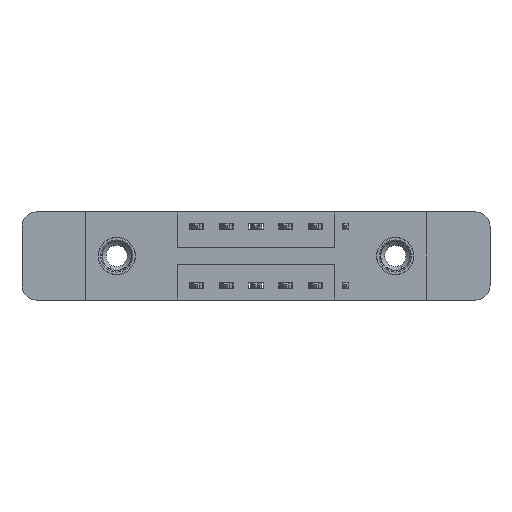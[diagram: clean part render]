
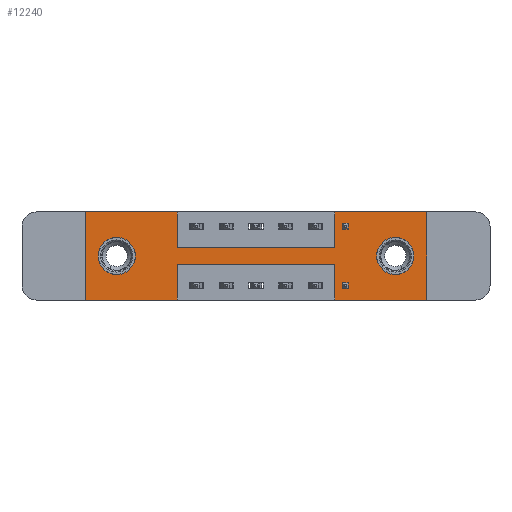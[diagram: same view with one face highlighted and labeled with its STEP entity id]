
A CAD part, front view. The second image highlights one B-rep face of the part: STEP entity #12240.
In plain terms, the highlighted planar face has unit normal (0, -1, 0).
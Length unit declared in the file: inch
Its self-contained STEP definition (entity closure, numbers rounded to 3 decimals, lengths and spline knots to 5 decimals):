
#74 = EDGE_CURVE ( 'NONE', #13054, #4540, #6638, .T. ) ;
#94 = DIRECTION ( 'NONE',  ( 0., 1., 0. ) ) ;
#152 = VECTOR ( 'NONE', #12726, 39.37008 ) ;
#212 = EDGE_CURVE ( 'NONE', #2639, #922, #11114, .T. ) ;
#272 = CARTESIAN_POINT ( 'NONE',  ( 0.1325, 0., -0.185 ) ) ;
#595 = EDGE_CURVE ( 'NONE', #10649, #8934, #3560, .T. ) ;
#611 = CARTESIAN_POINT ( 'NONE',  ( 0., 0., 0. ) ) ;
#614 = VERTEX_POINT ( 'NONE', #12001 ) ;
#895 = VECTOR ( 'NONE', #10591, 39.37008 ) ;
#922 = VERTEX_POINT ( 'NONE', #11918 ) ;
#938 = LINE ( 'NONE', #1008, #13102 ) ;
#957 = ORIENTED_EDGE ( 'NONE', *, *, #212, .F. ) ;
#1008 = CARTESIAN_POINT ( 'NONE',  ( 0., 0., -0.37 ) ) ;
#1032 = CARTESIAN_POINT ( 'NONE',  ( 0., 0., 0. ) ) ;
#1251 = VERTEX_POINT ( 'NONE', #7436 ) ;
#1263 = CARTESIAN_POINT ( 'NONE',  ( 1.3025, 0., -0.107 ) ) ;
#1266 = VECTOR ( 'NONE', #9973, 39.37008 ) ;
#1365 = EDGE_LOOP ( 'NONE', ( #5945, #7739, #6471, #9340, #9083, #13688, #10177, #9714, #957, #5654, #2848, #6998 ) ) ;
#1368 = CARTESIAN_POINT ( 'NONE',  ( 1.0475, 0., -0.37 ) ) ;
#1430 = VECTOR ( 'NONE', #10830, 39.37008 ) ;
#1546 = VERTEX_POINT ( 'NONE', #3613 ) ;
#1588 = LINE ( 'NONE', #611, #12780 ) ;
#1657 = VERTEX_POINT ( 'NONE', #9528 ) ;
#1797 = CARTESIAN_POINT ( 'NONE',  ( 0.1325, 0., -0.185 ) ) ;
#1889 = VECTOR ( 'NONE', #8711, 39.37008 ) ;
#2035 = CARTESIAN_POINT ( 'NONE',  ( 1.435, 0., 0. ) ) ;
#2095 = DIRECTION ( 'NONE',  ( 0., 1., 0. ) ) ;
#2115 = CARTESIAN_POINT ( 'NONE',  ( 0.1325, 0., -0.107 ) ) ;
#2263 = CARTESIAN_POINT ( 'NONE',  ( 1.3025, 0., -0.185 ) ) ;
#2639 = VERTEX_POINT ( 'NONE', #9645 ) ;
#2668 = CARTESIAN_POINT ( 'NONE',  ( 0.3875, 0., 0. ) ) ;
#2753 = ORIENTED_EDGE ( 'NONE', *, *, #3424, .T. ) ;
#2848 = ORIENTED_EDGE ( 'NONE', *, *, #7975, .F. ) ;
#2986 = EDGE_CURVE ( 'NONE', #3276, #13054, #7422, .T. ) ;
#3036 = DIRECTION ( 'NONE',  ( 0., 0., -1. ) ) ;
#3227 = EDGE_CURVE ( 'NONE', #922, #9711, #8189, .T. ) ;
#3228 = ORIENTED_EDGE ( 'NONE', *, *, #595, .T. ) ;
#3232 = CIRCLE ( 'NONE', #11150, 0.078 ) ;
#3276 = VERTEX_POINT ( 'NONE', #13511 ) ;
#3424 = EDGE_CURVE ( 'NONE', #8934, #10649, #3232, .T. ) ;
#3425 = VECTOR ( 'NONE', #10187, 39.37008 ) ;
#3449 = LINE ( 'NONE', #1368, #1266 ) ;
#3459 = VECTOR ( 'NONE', #9108, 39.37008 ) ;
#3560 = CIRCLE ( 'NONE', #5368, 0.078 ) ;
#3613 = CARTESIAN_POINT ( 'NONE',  ( 0., 0., 0. ) ) ;
#3797 = CARTESIAN_POINT ( 'NONE',  ( 0.3875, 0., -0.37 ) ) ;
#3992 = CARTESIAN_POINT ( 'NONE',  ( 0., 0., -0.37 ) ) ;
#4233 = FACE_OUTER_BOUND ( 'NONE', #1365, .T. ) ;
#4243 = DIRECTION ( 'NONE',  ( 0., 1., 0. ) ) ;
#4268 = AXIS2_PLACEMENT_3D ( 'NONE', #5300, #13944, #3036 ) ;
#4409 = DIRECTION ( 'NONE',  ( 0., 0., 1. ) ) ;
#4533 = EDGE_CURVE ( 'NONE', #10818, #1251, #3449, .T. ) ;
#4540 = VERTEX_POINT ( 'NONE', #11102 ) ;
#4701 = EDGE_CURVE ( 'NONE', #9711, #3276, #8729, .T. ) ;
#5027 = EDGE_CURVE ( 'NONE', #5985, #614, #8697, .T. ) ;
#5098 = ORIENTED_EDGE ( 'NONE', *, *, #10751, .T. ) ;
#5289 = CARTESIAN_POINT ( 'NONE',  ( 1.3025, 0., -0.185 ) ) ;
#5300 = CARTESIAN_POINT ( 'NONE',  ( 0., 0., -0.37 ) ) ;
#5368 = AXIS2_PLACEMENT_3D ( 'NONE', #2263, #94, #10738 ) ;
#5402 = EDGE_LOOP ( 'NONE', ( #11335, #5098 ) ) ;
#5415 = EDGE_CURVE ( 'NONE', #1251, #9273, #6204, .T. ) ;
#5429 = VECTOR ( 'NONE', #12583, 39.37008 ) ;
#5654 = ORIENTED_EDGE ( 'NONE', *, *, #9923, .F. ) ;
#5876 = DIRECTION ( 'NONE',  ( 0., 0., 1. ) ) ;
#5945 = ORIENTED_EDGE ( 'NONE', *, *, #13605, .F. ) ;
#5985 = VERTEX_POINT ( 'NONE', #2115 ) ;
#6204 = LINE ( 'NONE', #10680, #152 ) ;
#6334 = DIRECTION ( 'NONE',  ( -1., 0., 0. ) ) ;
#6427 = FACE_BOUND ( 'NONE', #13412, .T. ) ;
#6471 = ORIENTED_EDGE ( 'NONE', *, *, #4533, .F. ) ;
#6638 = LINE ( 'NONE', #7777, #1430 ) ;
#6642 = VECTOR ( 'NONE', #13115, 39.37008 ) ;
#6843 = CARTESIAN_POINT ( 'NONE',  ( 1.0475, 0., -0.15 ) ) ;
#6906 = LINE ( 'NONE', #3797, #5429 ) ;
#6998 = ORIENTED_EDGE ( 'NONE', *, *, #11338, .F. ) ;
#7121 = VERTEX_POINT ( 'NONE', #11855 ) ;
#7188 = CARTESIAN_POINT ( 'NONE',  ( 0.3875, 0., -0.15 ) ) ;
#7422 = LINE ( 'NONE', #1032, #1889 ) ;
#7436 = CARTESIAN_POINT ( 'NONE',  ( 1.0475, 0., -0.22 ) ) ;
#7635 = DIRECTION ( 'NONE',  ( 0., 1., 0. ) ) ;
#7739 = ORIENTED_EDGE ( 'NONE', *, *, #5415, .F. ) ;
#7777 = CARTESIAN_POINT ( 'NONE',  ( 1.435, 0., 0. ) ) ;
#7975 = EDGE_CURVE ( 'NONE', #1657, #1546, #1588, .T. ) ;
#8075 = CIRCLE ( 'NONE', #8534, 0.078 ) ;
#8189 = LINE ( 'NONE', #7188, #3459 ) ;
#8270 = PLANE ( 'NONE',  #4268 ) ;
#8317 = CARTESIAN_POINT ( 'NONE',  ( 1.3025, 0., -0.263 ) ) ;
#8534 = AXIS2_PLACEMENT_3D ( 'NONE', #272, #2095, #4409 ) ;
#8694 = DIRECTION ( 'NONE',  ( 1., 0., 0. ) ) ;
#8697 = CIRCLE ( 'NONE', #11408, 0.078 ) ;
#8711 = DIRECTION ( 'NONE',  ( 1., 0., 0. ) ) ;
#8729 = LINE ( 'NONE', #13185, #6642 ) ;
#8934 = VERTEX_POINT ( 'NONE', #8317 ) ;
#9083 = ORIENTED_EDGE ( 'NONE', *, *, #74, .F. ) ;
#9108 = DIRECTION ( 'NONE',  ( 1., 0., 0. ) ) ;
#9273 = VERTEX_POINT ( 'NONE', #13457 ) ;
#9340 = ORIENTED_EDGE ( 'NONE', *, *, #12571, .F. ) ;
#9518 = LINE ( 'NONE', #3992, #895 ) ;
#9528 = CARTESIAN_POINT ( 'NONE',  ( 0., 0., -0.37 ) ) ;
#9645 = CARTESIAN_POINT ( 'NONE',  ( 0.3875, 0., 0. ) ) ;
#9711 = VERTEX_POINT ( 'NONE', #6843 ) ;
#9714 = ORIENTED_EDGE ( 'NONE', *, *, #3227, .F. ) ;
#9761 = CARTESIAN_POINT ( 'NONE',  ( 0., 0., 0. ) ) ;
#9923 = EDGE_CURVE ( 'NONE', #1546, #2639, #10820, .T. ) ;
#9973 = DIRECTION ( 'NONE',  ( 0., 0., 1. ) ) ;
#10177 = ORIENTED_EDGE ( 'NONE', *, *, #4701, .F. ) ;
#10187 = DIRECTION ( 'NONE',  ( 0., 0., -1. ) ) ;
#10284 = CARTESIAN_POINT ( 'NONE',  ( 1.0475, 0., -0.37 ) ) ;
#10591 = DIRECTION ( 'NONE',  ( -1., 0., 0. ) ) ;
#10616 = FACE_BOUND ( 'NONE', #5402, .T. ) ;
#10649 = VERTEX_POINT ( 'NONE', #1263 ) ;
#10680 = CARTESIAN_POINT ( 'NONE',  ( 0.3875, 0., -0.22 ) ) ;
#10738 = DIRECTION ( 'NONE',  ( 0., 0., -1. ) ) ;
#10746 = DIRECTION ( 'NONE',  ( 0., 0., -1. ) ) ;
#10751 = EDGE_CURVE ( 'NONE', #614, #5985, #8075, .T. ) ;
#10818 = VERTEX_POINT ( 'NONE', #10284 ) ;
#10820 = LINE ( 'NONE', #9761, #12436 ) ;
#10830 = DIRECTION ( 'NONE',  ( 0., 0., -1. ) ) ;
#11102 = CARTESIAN_POINT ( 'NONE',  ( 1.435, 0., -0.37 ) ) ;
#11114 = LINE ( 'NONE', #2668, #3425 ) ;
#11150 = AXIS2_PLACEMENT_3D ( 'NONE', #5289, #7635, #10746 ) ;
#11335 = ORIENTED_EDGE ( 'NONE', *, *, #5027, .T. ) ;
#11338 = EDGE_CURVE ( 'NONE', #7121, #1657, #9518, .T. ) ;
#11408 = AXIS2_PLACEMENT_3D ( 'NONE', #1797, #4243, #13883 ) ;
#11855 = CARTESIAN_POINT ( 'NONE',  ( 0.3875, 0., -0.37 ) ) ;
#11918 = CARTESIAN_POINT ( 'NONE',  ( 0.3875, 0., -0.15 ) ) ;
#12001 = CARTESIAN_POINT ( 'NONE',  ( 0.1325, 0., -0.263 ) ) ;
#12240 = ADVANCED_FACE ( 'NONE', ( #6427, #10616, #4233 ), #8270, .T. ) ;
#12436 = VECTOR ( 'NONE', #8694, 39.37008 ) ;
#12571 = EDGE_CURVE ( 'NONE', #4540, #10818, #938, .T. ) ;
#12583 = DIRECTION ( 'NONE',  ( 0., 0., -1. ) ) ;
#12726 = DIRECTION ( 'NONE',  ( -1., 0., 0. ) ) ;
#12780 = VECTOR ( 'NONE', #5876, 39.37008 ) ;
#13054 = VERTEX_POINT ( 'NONE', #2035 ) ;
#13102 = VECTOR ( 'NONE', #6334, 39.37008 ) ;
#13115 = DIRECTION ( 'NONE',  ( 0., 0., 1. ) ) ;
#13185 = CARTESIAN_POINT ( 'NONE',  ( 1.0475, 0., 0. ) ) ;
#13412 = EDGE_LOOP ( 'NONE', ( #3228, #2753 ) ) ;
#13457 = CARTESIAN_POINT ( 'NONE',  ( 0.3875, 0., -0.22 ) ) ;
#13511 = CARTESIAN_POINT ( 'NONE',  ( 1.0475, 0., 0. ) ) ;
#13605 = EDGE_CURVE ( 'NONE', #9273, #7121, #6906, .T. ) ;
#13688 = ORIENTED_EDGE ( 'NONE', *, *, #2986, .F. ) ;
#13883 = DIRECTION ( 'NONE',  ( 0., 0., 1. ) ) ;
#13944 = DIRECTION ( 'NONE',  ( 0., -1., 0. ) ) ;
